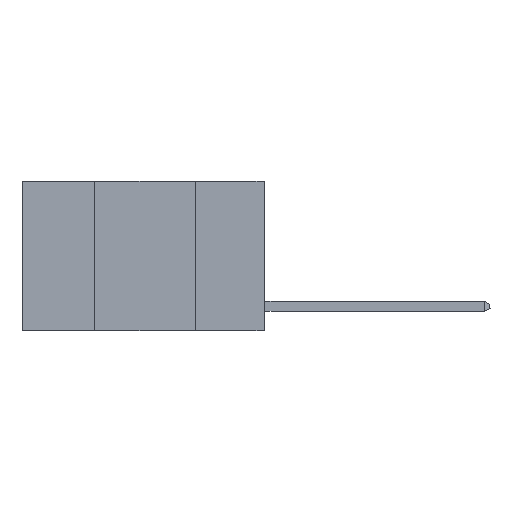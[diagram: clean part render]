
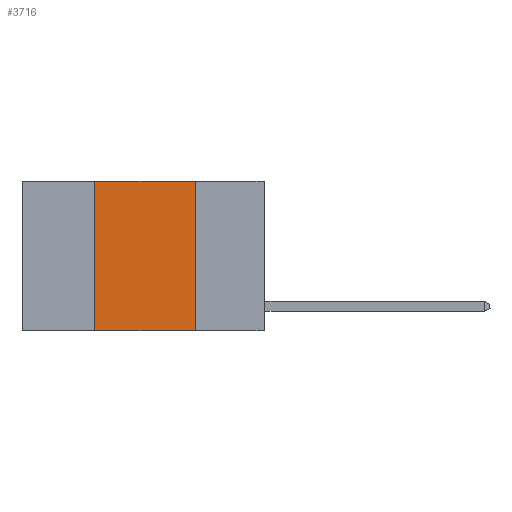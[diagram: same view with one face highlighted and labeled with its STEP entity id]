
A CAD part, left-side view. The second image highlights one B-rep face of the part: STEP entity #3716.
In plain terms, the highlighted planar face has unit normal (-1, 0, 0).
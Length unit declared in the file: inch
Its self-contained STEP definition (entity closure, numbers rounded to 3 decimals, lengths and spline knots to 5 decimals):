
#390 = LINE ( 'NONE', #4546, #5008 ) ;
#728 = EDGE_LOOP ( 'NONE', ( #7948, #4094, #2492, #2165 ) ) ;
#770 = FACE_OUTER_BOUND ( 'NONE', #728, .T. ) ;
#1887 = DIRECTION ( 'NONE',  ( 0., -1., 0. ) ) ;
#2139 = LINE ( 'NONE', #5709, #9044 ) ;
#2165 = ORIENTED_EDGE ( 'NONE', *, *, #4894, .T. ) ;
#2492 = ORIENTED_EDGE ( 'NONE', *, *, #4411, .F. ) ;
#2540 = EDGE_CURVE ( 'NONE', #6579, #6792, #390, .T. ) ;
#3023 = DIRECTION ( 'NONE',  ( 1., 0., 0. ) ) ;
#3034 = LINE ( 'NONE', #3722, #4292 ) ;
#3698 = CARTESIAN_POINT ( 'NONE',  ( 0., 0.42, -0.37 ) ) ;
#3716 = ADVANCED_FACE ( 'NONE', ( #770 ), #8044, .F. ) ;
#3722 = CARTESIAN_POINT ( 'NONE',  ( 0., 0.6, -0.37 ) ) ;
#3900 = DIRECTION ( 'NONE',  ( 0., 0., -1. ) ) ;
#4094 = ORIENTED_EDGE ( 'NONE', *, *, #5165, .F. ) ;
#4292 = VECTOR ( 'NONE', #6609, 39.37008 ) ;
#4411 = EDGE_CURVE ( 'NONE', #7105, #9218, #2139, .T. ) ;
#4546 = CARTESIAN_POINT ( 'NONE',  ( 0., 0.17, 0. ) ) ;
#4894 = EDGE_CURVE ( 'NONE', #7105, #6792, #3034, .T. ) ;
#5008 = VECTOR ( 'NONE', #3900, 39.37008 ) ;
#5165 = EDGE_CURVE ( 'NONE', #9218, #6579, #5415, .T. ) ;
#5415 = LINE ( 'NONE', #8276, #6197 ) ;
#5709 = CARTESIAN_POINT ( 'NONE',  ( 0., 0.42, 0. ) ) ;
#5737 = CARTESIAN_POINT ( 'NONE',  ( 0., 0.6, 0. ) ) ;
#6197 = VECTOR ( 'NONE', #1887, 39.37008 ) ;
#6579 = VERTEX_POINT ( 'NONE', #7703 ) ;
#6609 = DIRECTION ( 'NONE',  ( 0., -1., 0. ) ) ;
#6792 = VERTEX_POINT ( 'NONE', #6819 ) ;
#6819 = CARTESIAN_POINT ( 'NONE',  ( 0., 0.17, -0.37 ) ) ;
#7105 = VERTEX_POINT ( 'NONE', #3698 ) ;
#7232 = DIRECTION ( 'NONE',  ( 0., 0., 1. ) ) ;
#7703 = CARTESIAN_POINT ( 'NONE',  ( 0., 0.17, 0. ) ) ;
#7948 = ORIENTED_EDGE ( 'NONE', *, *, #2540, .F. ) ;
#7956 = DIRECTION ( 'NONE',  ( 0., 0., -1. ) ) ;
#8044 = PLANE ( 'NONE',  #8051 ) ;
#8051 = AXIS2_PLACEMENT_3D ( 'NONE', #5737, #3023, #7956 ) ;
#8276 = CARTESIAN_POINT ( 'NONE',  ( 0., 0.6, 0. ) ) ;
#8751 = CARTESIAN_POINT ( 'NONE',  ( 0., 0.42, 0. ) ) ;
#9044 = VECTOR ( 'NONE', #7232, 39.37008 ) ;
#9218 = VERTEX_POINT ( 'NONE', #8751 ) ;
